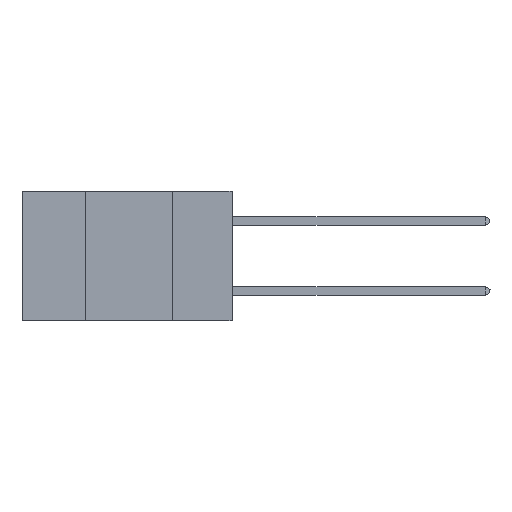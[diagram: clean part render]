
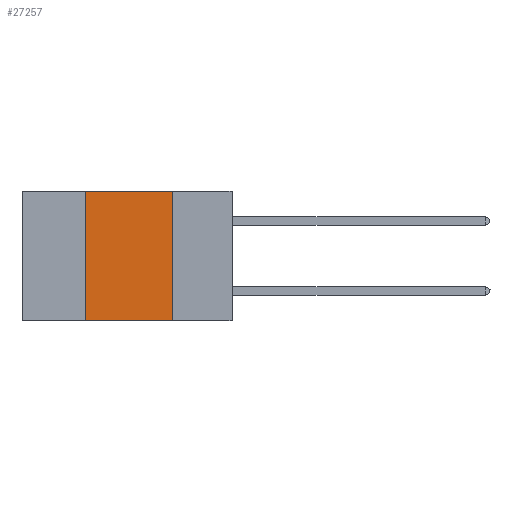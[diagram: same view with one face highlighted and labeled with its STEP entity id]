
A CAD part, left-side view. The second image highlights one B-rep face of the part: STEP entity #27257.
In plain terms, the highlighted planar face has unit normal (-1, 0, 0).
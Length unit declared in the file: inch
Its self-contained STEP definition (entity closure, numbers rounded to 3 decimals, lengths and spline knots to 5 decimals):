
#95 = CARTESIAN_POINT ( 'NONE',  ( 0., 0.42, 0. ) ) ;
#741 = EDGE_LOOP ( 'NONE', ( #8355, #14638, #6289, #15666 ) ) ;
#1447 = LINE ( 'NONE', #13272, #11657 ) ;
#1523 = VERTEX_POINT ( 'NONE', #11844 ) ;
#2256 = CARTESIAN_POINT ( 'NONE',  ( 0., 0.42, 0. ) ) ;
#2511 = CARTESIAN_POINT ( 'NONE',  ( 0., 0.17, 0. ) ) ;
#5752 = DIRECTION ( 'NONE',  ( 0., 0., -1. ) ) ;
#6109 = VECTOR ( 'NONE', #25256, 39.37008 ) ;
#6289 = ORIENTED_EDGE ( 'NONE', *, *, #22502, .F. ) ;
#7531 = VERTEX_POINT ( 'NONE', #13322 ) ;
#8355 = ORIENTED_EDGE ( 'NONE', *, *, #18552, .F. ) ;
#8985 = FACE_OUTER_BOUND ( 'NONE', #741, .T. ) ;
#9056 = DIRECTION ( 'NONE',  ( 0., -1., 0. ) ) ;
#9210 = CARTESIAN_POINT ( 'NONE',  ( 0., 0.6, -0.37 ) ) ;
#10319 = VECTOR ( 'NONE', #9056, 39.37008 ) ;
#11408 = EDGE_CURVE ( 'NONE', #17100, #13126, #15748, .T. ) ;
#11657 = VECTOR ( 'NONE', #5752, 39.37008 ) ;
#11765 = DIRECTION ( 'NONE',  ( 0., 0., 1. ) ) ;
#11844 = CARTESIAN_POINT ( 'NONE',  ( 0., 0.17, -0.37 ) ) ;
#12410 = AXIS2_PLACEMENT_3D ( 'NONE', #13441, #13135, #27381 ) ;
#13126 = VERTEX_POINT ( 'NONE', #2511 ) ;
#13135 = DIRECTION ( 'NONE',  ( 1., 0., 0. ) ) ;
#13272 = CARTESIAN_POINT ( 'NONE',  ( 0., 0.17, 0. ) ) ;
#13322 = CARTESIAN_POINT ( 'NONE',  ( 0., 0.42, -0.37 ) ) ;
#13441 = CARTESIAN_POINT ( 'NONE',  ( 0., 0.6, 0. ) ) ;
#14638 = ORIENTED_EDGE ( 'NONE', *, *, #11408, .F. ) ;
#15666 = ORIENTED_EDGE ( 'NONE', *, *, #23875, .T. ) ;
#15748 = LINE ( 'NONE', #16061, #6109 ) ;
#16061 = CARTESIAN_POINT ( 'NONE',  ( 0., 0.6, 0. ) ) ;
#17100 = VERTEX_POINT ( 'NONE', #95 ) ;
#18183 = PLANE ( 'NONE',  #12410 ) ;
#18552 = EDGE_CURVE ( 'NONE', #13126, #1523, #1447, .T. ) ;
#22070 = VECTOR ( 'NONE', #11765, 39.37008 ) ;
#22502 = EDGE_CURVE ( 'NONE', #7531, #17100, #23273, .T. ) ;
#23273 = LINE ( 'NONE', #2256, #22070 ) ;
#23875 = EDGE_CURVE ( 'NONE', #7531, #1523, #25757, .T. ) ;
#25256 = DIRECTION ( 'NONE',  ( 0., -1., 0. ) ) ;
#25757 = LINE ( 'NONE', #9210, #10319 ) ;
#27257 = ADVANCED_FACE ( 'NONE', ( #8985 ), #18183, .F. ) ;
#27381 = DIRECTION ( 'NONE',  ( 0., 0., -1. ) ) ;
